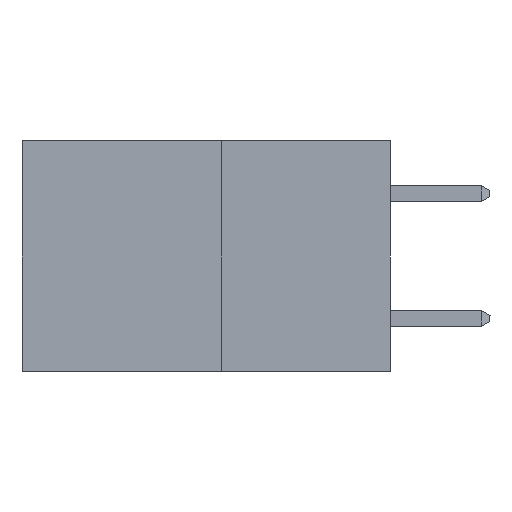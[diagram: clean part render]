
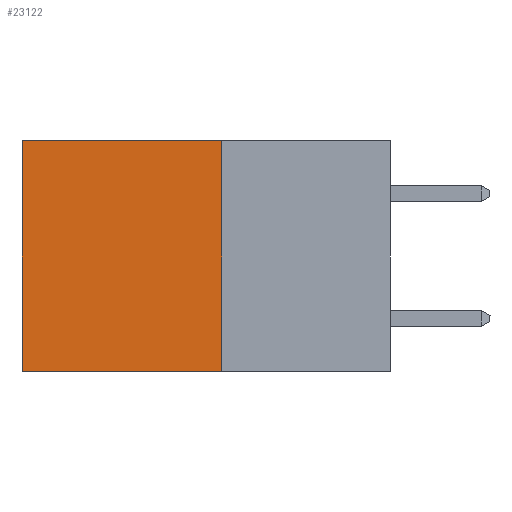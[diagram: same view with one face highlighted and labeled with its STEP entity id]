
A CAD part, left-side view. The second image highlights one B-rep face of the part: STEP entity #23122.
In plain terms, the highlighted planar face has unit normal (-1, 0, 0).
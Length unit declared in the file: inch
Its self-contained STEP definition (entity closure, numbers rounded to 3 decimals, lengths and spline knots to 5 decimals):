
#101 = ORIENTED_EDGE ( 'NONE', *, *, #15270, .T. ) ;
#740 = EDGE_CURVE ( 'NONE', #30018, #24068, #12369, .T. ) ;
#1729 = CARTESIAN_POINT ( 'NONE',  ( 0.277, 0.27, -0.37 ) ) ;
#1855 = VECTOR ( 'NONE', #22087, 39.37008 ) ;
#2017 = LINE ( 'NONE', #16925, #26150 ) ;
#2938 = VERTEX_POINT ( 'NONE', #23150 ) ;
#2996 = ORIENTED_EDGE ( 'NONE', *, *, #20580, .T. ) ;
#5382 = VECTOR ( 'NONE', #27220, 39.37008 ) ;
#6759 = CARTESIAN_POINT ( 'NONE',  ( 0.277, 0.27, -0.37 ) ) ;
#11501 = EDGE_CURVE ( 'NONE', #2938, #30018, #20547, .T. ) ;
#12369 = LINE ( 'NONE', #15161, #5382 ) ;
#12794 = CARTESIAN_POINT ( 'NONE',  ( 0.277, 0.27, -0.37 ) ) ;
#12977 = LINE ( 'NONE', #30081, #25369 ) ;
#15161 = CARTESIAN_POINT ( 'NONE',  ( 0.277, 0.27, -0.37 ) ) ;
#15270 = EDGE_CURVE ( 'NONE', #2938, #21495, #12977, .T. ) ;
#15689 = CARTESIAN_POINT ( 'NONE',  ( 0.277, 0.59, 0. ) ) ;
#15897 = DIRECTION ( 'NONE',  ( 0., 0., -1. ) ) ;
#16237 = DIRECTION ( 'NONE',  ( 0., 1., 0. ) ) ;
#16925 = CARTESIAN_POINT ( 'NONE',  ( 0.277, 0.59, -0.37 ) ) ;
#17018 = FACE_OUTER_BOUND ( 'NONE', #25673, .T. ) ;
#17687 = ORIENTED_EDGE ( 'NONE', *, *, #740, .F. ) ;
#18989 = CARTESIAN_POINT ( 'NONE',  ( 0.277, 0.59, -0.37 ) ) ;
#19269 = DIRECTION ( 'NONE',  ( 0., 0., -1. ) ) ;
#20547 = LINE ( 'NONE', #12794, #1855 ) ;
#20580 = EDGE_CURVE ( 'NONE', #21495, #24068, #2017, .T. ) ;
#21495 = VERTEX_POINT ( 'NONE', #15689 ) ;
#22087 = DIRECTION ( 'NONE',  ( 0., 0., -1. ) ) ;
#23122 = ADVANCED_FACE ( 'NONE', ( #17018 ), #25152, .F. ) ;
#23150 = CARTESIAN_POINT ( 'NONE',  ( 0.277, 0.27, 0. ) ) ;
#23906 = AXIS2_PLACEMENT_3D ( 'NONE', #1729, #29752, #15897 ) ;
#24068 = VERTEX_POINT ( 'NONE', #18989 ) ;
#25152 = PLANE ( 'NONE',  #23906 ) ;
#25369 = VECTOR ( 'NONE', #16237, 39.37008 ) ;
#25673 = EDGE_LOOP ( 'NONE', ( #2996, #17687, #28950, #101 ) ) ;
#26150 = VECTOR ( 'NONE', #19269, 39.37008 ) ;
#27220 = DIRECTION ( 'NONE',  ( 0., 1., 0. ) ) ;
#28950 = ORIENTED_EDGE ( 'NONE', *, *, #11501, .F. ) ;
#29752 = DIRECTION ( 'NONE',  ( 1., 0., 0. ) ) ;
#30018 = VERTEX_POINT ( 'NONE', #6759 ) ;
#30081 = CARTESIAN_POINT ( 'NONE',  ( 0.277, 0.27, 0. ) ) ;
